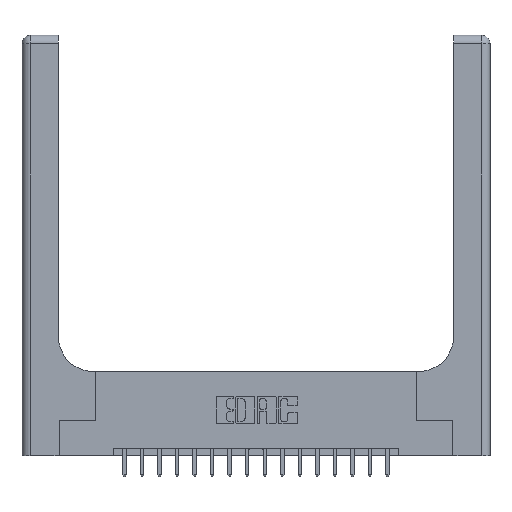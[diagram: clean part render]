
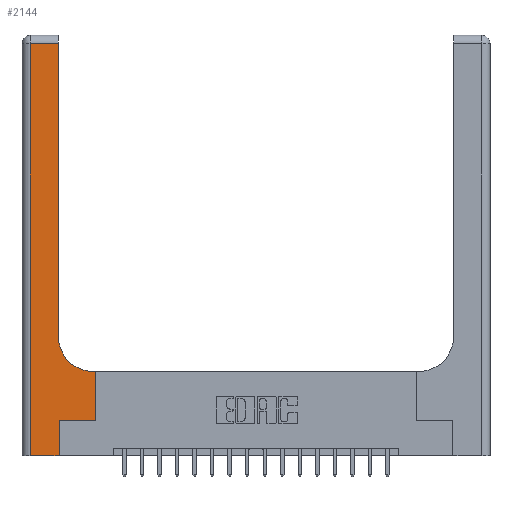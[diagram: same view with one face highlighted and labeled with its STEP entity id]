
A CAD part, top view. The second image highlights one B-rep face of the part: STEP entity #2144.
In plain terms, the highlighted planar face has unit normal (0, 0, 1).
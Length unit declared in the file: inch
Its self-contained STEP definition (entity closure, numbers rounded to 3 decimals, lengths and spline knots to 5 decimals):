
#31 = ORIENTED_EDGE ( 'NONE', *, *, #6348, .T. ) ;
#137 = VECTOR ( 'NONE', #11843, 39.37008 ) ;
#194 = EDGE_CURVE ( 'NONE', #3455, #15337, #7571, .T. ) ;
#1172 = LINE ( 'NONE', #18628, #2579 ) ;
#1946 = PLANE ( 'NONE',  #11573 ) ;
#2088 = VERTEX_POINT ( 'NONE', #2205 ) ;
#2090 = DIRECTION ( 'NONE',  ( 0., 0., -1. ) ) ;
#2144 = ADVANCED_FACE ( 'NONE', ( #4486 ), #1946, .F. ) ;
#2205 = CARTESIAN_POINT ( 'NONE',  ( 0.528, 0.25, 0.37 ) ) ;
#2579 = VECTOR ( 'NONE', #11252, 39.37008 ) ;
#2684 = VERTEX_POINT ( 'NONE', #13851 ) ;
#2917 = CARTESIAN_POINT ( 'NONE',  ( 0.26, 3., 0.37 ) ) ;
#3332 = EDGE_CURVE ( 'NONE', #17088, #3462, #10100, .T. ) ;
#3410 = LINE ( 'NONE', #4428, #9592 ) ;
#3455 = VERTEX_POINT ( 'NONE', #8217 ) ;
#3462 = VERTEX_POINT ( 'NONE', #9548 ) ;
#3695 = DIRECTION ( 'NONE',  ( 0., 1., 0. ) ) ;
#3944 = ORIENTED_EDGE ( 'NONE', *, *, #3332, .T. ) ;
#4306 = ORIENTED_EDGE ( 'NONE', *, *, #4519, .T. ) ;
#4324 = ORIENTED_EDGE ( 'NONE', *, *, #17290, .T. ) ;
#4428 = CARTESIAN_POINT ( 'NONE',  ( 0.06, 3., 0.37 ) ) ;
#4486 = FACE_OUTER_BOUND ( 'NONE', #13878, .T. ) ;
#4519 = EDGE_CURVE ( 'NONE', #13407, #9954, #6325, .T. ) ;
#4841 = DIRECTION ( 'NONE',  ( 0., 0., -1. ) ) ;
#5233 = CIRCLE ( 'NONE', #17327, 0.25 ) ;
#5436 = CARTESIAN_POINT ( 'NONE',  ( 0.528, 0.6, 0.37 ) ) ;
#5831 = VECTOR ( 'NONE', #14823, 39.37008 ) ;
#6325 = LINE ( 'NONE', #14120, #6782 ) ;
#6348 = EDGE_CURVE ( 'NONE', #2684, #13407, #1172, .T. ) ;
#6400 = CARTESIAN_POINT ( 'NONE',  ( 0., 3., 0.37 ) ) ;
#6723 = DIRECTION ( 'NONE',  ( -1., 0., 0. ) ) ;
#6779 = CARTESIAN_POINT ( 'NONE',  ( 0.26, 2.94, 0.37 ) ) ;
#6782 = VECTOR ( 'NONE', #10928, 39.37008 ) ;
#7259 = ORIENTED_EDGE ( 'NONE', *, *, #13038, .T. ) ;
#7571 = LINE ( 'NONE', #2917, #18899 ) ;
#8217 = CARTESIAN_POINT ( 'NONE',  ( 0.26, 0.85, 0.37 ) ) ;
#8572 = CARTESIAN_POINT ( 'NONE',  ( 0.265, 0.25, 0.37 ) ) ;
#9141 = CARTESIAN_POINT ( 'NONE',  ( 0.06, 2.94, 0.37 ) ) ;
#9548 = CARTESIAN_POINT ( 'NONE',  ( 0.51, 0.6, 0.37 ) ) ;
#9592 = VECTOR ( 'NONE', #10205, 39.37008 ) ;
#9856 = VECTOR ( 'NONE', #3695, 39.37008 ) ;
#9954 = VERTEX_POINT ( 'NONE', #8572 ) ;
#9991 = ORIENTED_EDGE ( 'NONE', *, *, #15753, .T. ) ;
#10000 = EDGE_CURVE ( 'NONE', #15111, #2684, #3410, .T. ) ;
#10100 = LINE ( 'NONE', #13357, #137 ) ;
#10205 = DIRECTION ( 'NONE',  ( 0., -1., 0. ) ) ;
#10777 = DIRECTION ( 'NONE',  ( 1., 0., 0. ) ) ;
#10928 = DIRECTION ( 'NONE',  ( 0., 1., 0. ) ) ;
#11252 = DIRECTION ( 'NONE',  ( 1., 0., 0. ) ) ;
#11573 = AXIS2_PLACEMENT_3D ( 'NONE', #6400, #2090, #6723 ) ;
#11843 = DIRECTION ( 'NONE',  ( -1., 0., 0. ) ) ;
#12098 = CARTESIAN_POINT ( 'NONE',  ( 0., 2.94, 0.37 ) ) ;
#13038 = EDGE_CURVE ( 'NONE', #3462, #3455, #5233, .T. ) ;
#13045 = LINE ( 'NONE', #14625, #5831 ) ;
#13276 = VECTOR ( 'NONE', #18225, 39.37008 ) ;
#13357 = CARTESIAN_POINT ( 'NONE',  ( 0.26, 0.6, 0.37 ) ) ;
#13407 = VERTEX_POINT ( 'NONE', #15678 ) ;
#13538 = DIRECTION ( 'NONE',  ( 0., 1., 0. ) ) ;
#13776 = EDGE_CURVE ( 'NONE', #2088, #17088, #15845, .T. ) ;
#13851 = CARTESIAN_POINT ( 'NONE',  ( 0.06, 0., 0.37 ) ) ;
#13878 = EDGE_LOOP ( 'NONE', ( #15719, #9991, #17319, #31, #4306, #4324, #16546, #3944, #7259 ) ) ;
#14120 = CARTESIAN_POINT ( 'NONE',  ( 0.265, 0., 0.37 ) ) ;
#14625 = CARTESIAN_POINT ( 'NONE',  ( 0.265, 0.25, 0.37 ) ) ;
#14823 = DIRECTION ( 'NONE',  ( 1., 0., 0. ) ) ;
#15111 = VERTEX_POINT ( 'NONE', #9141 ) ;
#15337 = VERTEX_POINT ( 'NONE', #6779 ) ;
#15678 = CARTESIAN_POINT ( 'NONE',  ( 0.265, 0., 0.37 ) ) ;
#15710 = CARTESIAN_POINT ( 'NONE',  ( 0.528, 0.25, 0.37 ) ) ;
#15719 = ORIENTED_EDGE ( 'NONE', *, *, #194, .T. ) ;
#15753 = EDGE_CURVE ( 'NONE', #15337, #15111, #17156, .T. ) ;
#15845 = LINE ( 'NONE', #15710, #9856 ) ;
#16398 = CARTESIAN_POINT ( 'NONE',  ( 0.51, 0.85, 0.37 ) ) ;
#16546 = ORIENTED_EDGE ( 'NONE', *, *, #13776, .T. ) ;
#17088 = VERTEX_POINT ( 'NONE', #5436 ) ;
#17156 = LINE ( 'NONE', #12098, #13276 ) ;
#17290 = EDGE_CURVE ( 'NONE', #9954, #2088, #13045, .T. ) ;
#17319 = ORIENTED_EDGE ( 'NONE', *, *, #10000, .T. ) ;
#17327 = AXIS2_PLACEMENT_3D ( 'NONE', #16398, #4841, #10777 ) ;
#18225 = DIRECTION ( 'NONE',  ( -1., 0., 0. ) ) ;
#18628 = CARTESIAN_POINT ( 'NONE',  ( 0., 0., 0.37 ) ) ;
#18899 = VECTOR ( 'NONE', #13538, 39.37008 ) ;
